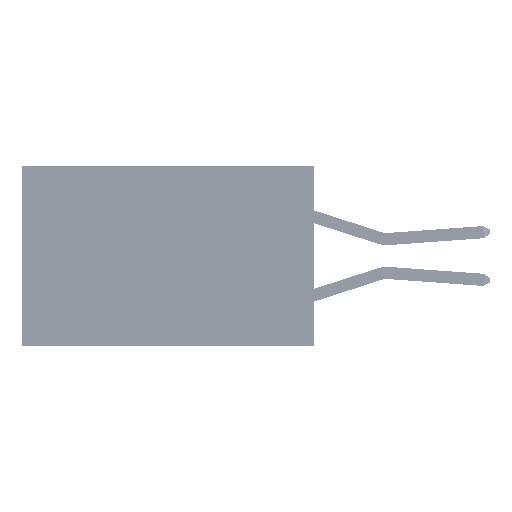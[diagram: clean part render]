
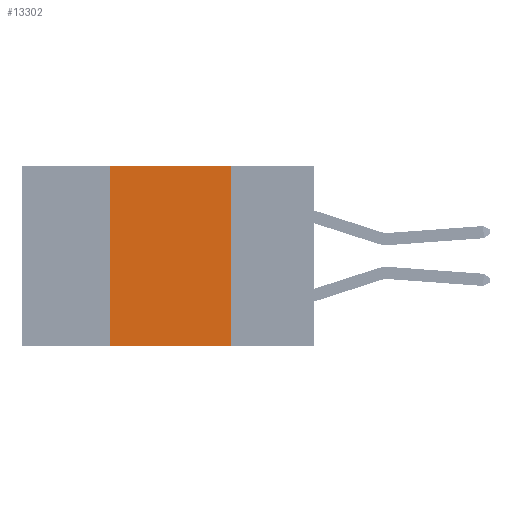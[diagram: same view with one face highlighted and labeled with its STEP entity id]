
A CAD part, left-side view. The second image highlights one B-rep face of the part: STEP entity #13302.
In plain terms, the highlighted planar face has unit normal (-1, 0, 0).
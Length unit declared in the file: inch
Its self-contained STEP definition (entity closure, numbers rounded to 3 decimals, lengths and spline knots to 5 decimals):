
#536 = ORIENTED_EDGE ( 'NONE', *, *, #9180, .F. ) ;
#1223 = DIRECTION ( 'NONE',  ( 0., 0., 1. ) ) ;
#1717 = EDGE_CURVE ( 'NONE', #4763, #11206, #21757, .T. ) ;
#1752 = CARTESIAN_POINT ( 'NONE',  ( 0., 0.17, 0. ) ) ;
#2023 = CARTESIAN_POINT ( 'NONE',  ( 0., 0.6, -0.37 ) ) ;
#4763 = VERTEX_POINT ( 'NONE', #40888 ) ;
#5087 = VERTEX_POINT ( 'NONE', #1752 ) ;
#5148 = DIRECTION ( 'NONE',  ( 0., 0., -1. ) ) ;
#7343 = EDGE_LOOP ( 'NONE', ( #536, #11853, #26961, #34409 ) ) ;
#9180 = EDGE_CURVE ( 'NONE', #5087, #19631, #37524, .T. ) ;
#9517 = CARTESIAN_POINT ( 'NONE',  ( 0., 0.17, 0. ) ) ;
#11206 = VERTEX_POINT ( 'NONE', #30537 ) ;
#11830 = VECTOR ( 'NONE', #1223, 39.37008 ) ;
#11853 = ORIENTED_EDGE ( 'NONE', *, *, #35588, .F. ) ;
#12429 = LINE ( 'NONE', #2023, #20014 ) ;
#13302 = ADVANCED_FACE ( 'NONE', ( #27289 ), #23766, .F. ) ;
#18367 = EDGE_CURVE ( 'NONE', #4763, #19631, #12429, .T. ) ;
#19631 = VERTEX_POINT ( 'NONE', #47610 ) ;
#20014 = VECTOR ( 'NONE', #31880, 39.37008 ) ;
#21757 = LINE ( 'NONE', #27248, #11830 ) ;
#23766 = PLANE ( 'NONE',  #26635 ) ;
#25162 = LINE ( 'NONE', #45895, #44629 ) ;
#26635 = AXIS2_PLACEMENT_3D ( 'NONE', #34723, #27472, #5148 ) ;
#26961 = ORIENTED_EDGE ( 'NONE', *, *, #1717, .F. ) ;
#27248 = CARTESIAN_POINT ( 'NONE',  ( 0., 0.42, 0. ) ) ;
#27289 = FACE_OUTER_BOUND ( 'NONE', #7343, .T. ) ;
#27472 = DIRECTION ( 'NONE',  ( 1., 0., 0. ) ) ;
#30537 = CARTESIAN_POINT ( 'NONE',  ( 0., 0.42, 0. ) ) ;
#31880 = DIRECTION ( 'NONE',  ( 0., -1., 0. ) ) ;
#34409 = ORIENTED_EDGE ( 'NONE', *, *, #18367, .T. ) ;
#34723 = CARTESIAN_POINT ( 'NONE',  ( 0., 0.6, 0. ) ) ;
#34898 = DIRECTION ( 'NONE',  ( 0., -1., 0. ) ) ;
#35588 = EDGE_CURVE ( 'NONE', #11206, #5087, #25162, .T. ) ;
#37524 = LINE ( 'NONE', #9517, #46068 ) ;
#40888 = CARTESIAN_POINT ( 'NONE',  ( 0., 0.42, -0.37 ) ) ;
#42633 = DIRECTION ( 'NONE',  ( 0., 0., -1. ) ) ;
#44629 = VECTOR ( 'NONE', #34898, 39.37008 ) ;
#45895 = CARTESIAN_POINT ( 'NONE',  ( 0., 0.6, 0. ) ) ;
#46068 = VECTOR ( 'NONE', #42633, 39.37008 ) ;
#47610 = CARTESIAN_POINT ( 'NONE',  ( 0., 0.17, -0.37 ) ) ;
